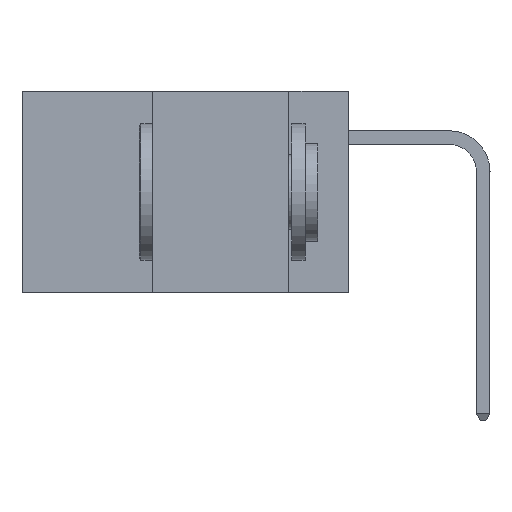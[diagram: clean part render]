
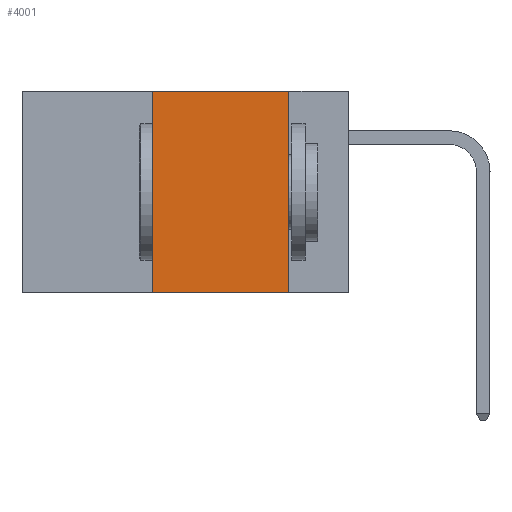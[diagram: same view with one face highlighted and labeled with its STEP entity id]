
A CAD part, left-side view. The second image highlights one B-rep face of the part: STEP entity #4001.
In plain terms, the highlighted planar face has unit normal (-1, 0, 0).
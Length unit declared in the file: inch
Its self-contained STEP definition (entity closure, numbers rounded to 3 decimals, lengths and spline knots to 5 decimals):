
#1292 = ORIENTED_EDGE ( 'NONE', *, *, #2742, .F. ) ;
#2742 = EDGE_CURVE ( 'NONE', #13243, #10812, #3342, .T. ) ;
#3114 = CARTESIAN_POINT ( 'NONE',  ( 0., 0.36, 0. ) ) ;
#3342 = LINE ( 'NONE', #31169, #30416 ) ;
#4001 = ADVANCED_FACE ( 'NONE', ( #32778 ), #27215, .F. ) ;
#4459 = ORIENTED_EDGE ( 'NONE', *, *, #12173, .F. ) ;
#5522 = VECTOR ( 'NONE', #8708, 39.37008 ) ;
#8708 = DIRECTION ( 'NONE',  ( 0., -1., 0. ) ) ;
#10812 = VERTEX_POINT ( 'NONE', #29006 ) ;
#10882 = CARTESIAN_POINT ( 'NONE',  ( 0., 0.11, 0. ) ) ;
#11024 = CARTESIAN_POINT ( 'NONE',  ( 0., 0.6, 0. ) ) ;
#11300 = CARTESIAN_POINT ( 'NONE',  ( 0., 0.6, -0.37 ) ) ;
#12173 = EDGE_CURVE ( 'NONE', #34055, #13243, #20355, .T. ) ;
#13090 = ORIENTED_EDGE ( 'NONE', *, *, #25565, .F. ) ;
#13243 = VERTEX_POINT ( 'NONE', #3114 ) ;
#13749 = DIRECTION ( 'NONE',  ( 1., 0., 0. ) ) ;
#13946 = VERTEX_POINT ( 'NONE', #27668 ) ;
#17006 = CARTESIAN_POINT ( 'NONE',  ( 0., 0.36, 0. ) ) ;
#19326 = CARTESIAN_POINT ( 'NONE',  ( 0., 0.36, -0.37 ) ) ;
#20355 = LINE ( 'NONE', #17006, #26693 ) ;
#20616 = AXIS2_PLACEMENT_3D ( 'NONE', #11024, #13749, #32586 ) ;
#22509 = DIRECTION ( 'NONE',  ( 0., 0., 1. ) ) ;
#24396 = DIRECTION ( 'NONE',  ( 0., -1., 0. ) ) ;
#24450 = EDGE_CURVE ( 'NONE', #34055, #13946, #34142, .T. ) ;
#24752 = ORIENTED_EDGE ( 'NONE', *, *, #24450, .T. ) ;
#25565 = EDGE_CURVE ( 'NONE', #10812, #13946, #32384, .T. ) ;
#26693 = VECTOR ( 'NONE', #22509, 39.37008 ) ;
#27215 = PLANE ( 'NONE',  #20616 ) ;
#27668 = CARTESIAN_POINT ( 'NONE',  ( 0., 0.11, -0.37 ) ) ;
#29006 = CARTESIAN_POINT ( 'NONE',  ( 0., 0.11, 0. ) ) ;
#29792 = DIRECTION ( 'NONE',  ( 0., 0., -1. ) ) ;
#30416 = VECTOR ( 'NONE', #24396, 39.37008 ) ;
#31169 = CARTESIAN_POINT ( 'NONE',  ( 0., 0.6, 0. ) ) ;
#31570 = VECTOR ( 'NONE', #29792, 39.37008 ) ;
#32384 = LINE ( 'NONE', #10882, #31570 ) ;
#32586 = DIRECTION ( 'NONE',  ( 0., 0., -1. ) ) ;
#32778 = FACE_OUTER_BOUND ( 'NONE', #33386, .T. ) ;
#33386 = EDGE_LOOP ( 'NONE', ( #13090, #1292, #4459, #24752 ) ) ;
#34055 = VERTEX_POINT ( 'NONE', #19326 ) ;
#34142 = LINE ( 'NONE', #11300, #5522 ) ;
